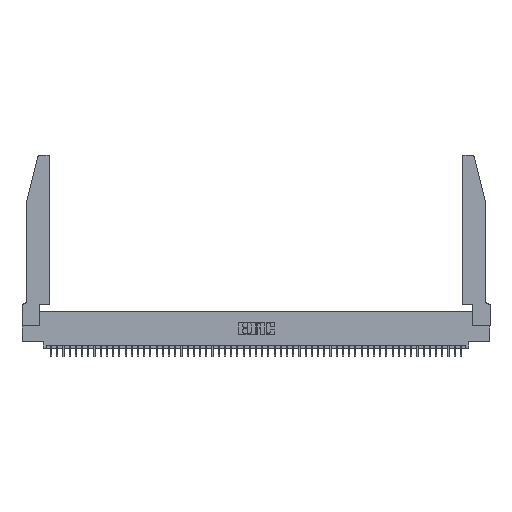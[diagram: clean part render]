
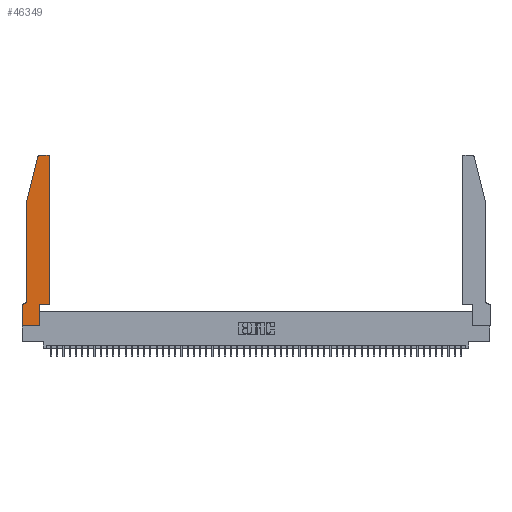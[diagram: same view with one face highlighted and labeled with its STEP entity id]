
A CAD part, top view. The second image highlights one B-rep face of the part: STEP entity #46349.
In plain terms, the highlighted planar face has unit normal (0, 0, 1).
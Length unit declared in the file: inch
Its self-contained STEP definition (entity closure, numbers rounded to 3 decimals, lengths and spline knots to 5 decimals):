
#255 = EDGE_CURVE ( 'NONE', #29158, #11118, #25259, .T. ) ;
#422 = DIRECTION ( 'NONE',  ( 0., 1., 0. ) ) ;
#855 = CARTESIAN_POINT ( 'NONE',  ( 0., 0.35, 0.37 ) ) ;
#1293 = VECTOR ( 'NONE', #41936, 39.37008 ) ;
#1744 = LINE ( 'NONE', #14056, #22702 ) ;
#2047 = ORIENTED_EDGE ( 'NONE', *, *, #10825, .T. ) ;
#2261 = VECTOR ( 'NONE', #49794, 39.37008 ) ;
#2536 = EDGE_CURVE ( 'NONE', #11118, #16320, #14779, .T. ) ;
#3194 = LINE ( 'NONE', #44871, #2261 ) ;
#4353 = VERTEX_POINT ( 'NONE', #20992 ) ;
#4741 = DIRECTION ( 'NONE',  ( 1., 0., 0. ) ) ;
#5598 = LINE ( 'NONE', #26940, #16897 ) ;
#6244 = LINE ( 'NONE', #31736, #15475 ) ;
#6342 = AXIS2_PLACEMENT_3D ( 'NONE', #29683, #42881, #47290 ) ;
#6368 = EDGE_CURVE ( 'NONE', #54025, #15663, #5598, .T. ) ;
#8783 = CARTESIAN_POINT ( 'NONE',  ( 0.2605, 2.75, 0.37 ) ) ;
#10032 = CARTESIAN_POINT ( 'NONE',  ( 0., 0.35, 0.37 ) ) ;
#10690 = AXIS2_PLACEMENT_3D ( 'NONE', #32336, #24099, #11267 ) ;
#10755 = CIRCLE ( 'NONE', #6342, 0.03 ) ;
#10825 = EDGE_CURVE ( 'NONE', #53074, #42692, #49253, .T. ) ;
#10941 = CARTESIAN_POINT ( 'NONE',  ( 0.0755, 0.42, 0.37 ) ) ;
#11118 = VERTEX_POINT ( 'NONE', #38383 ) ;
#11267 = DIRECTION ( 'NONE',  ( 1., 0., 0. ) ) ;
#11764 = ORIENTED_EDGE ( 'NONE', *, *, #50175, .T. ) ;
#12223 = CARTESIAN_POINT ( 'NONE',  ( 0.0755, 0.35, 0.37 ) ) ;
#13361 = VECTOR ( 'NONE', #422, 39.37008 ) ;
#13656 = ORIENTED_EDGE ( 'NONE', *, *, #39989, .T. ) ;
#13779 = DIRECTION ( 'NONE',  ( 0., -1., 0. ) ) ;
#14056 = CARTESIAN_POINT ( 'NONE',  ( 0.0755, 2., 0.37 ) ) ;
#14239 = CARTESIAN_POINT ( 'NONE',  ( 0.4505, 0.35, 0.37 ) ) ;
#14523 = EDGE_CURVE ( 'NONE', #15663, #51088, #3194, .T. ) ;
#14779 = LINE ( 'NONE', #14239, #26258 ) ;
#14914 = PLANE ( 'NONE',  #29344 ) ;
#15116 = DIRECTION ( 'NONE',  ( 0., 0., -1. ) ) ;
#15122 = CARTESIAN_POINT ( 'NONE',  ( 0.284, 2.75, 0.37 ) ) ;
#15475 = VECTOR ( 'NONE', #23750, 39.37008 ) ;
#15663 = VERTEX_POINT ( 'NONE', #17989 ) ;
#16306 = CARTESIAN_POINT ( 'NONE',  ( 0.0055, 0.35, 0.37 ) ) ;
#16320 = VERTEX_POINT ( 'NONE', #30706 ) ;
#16897 = VECTOR ( 'NONE', #27759, 39.37008 ) ;
#17989 = CARTESIAN_POINT ( 'NONE',  ( 0., 0., 0.37 ) ) ;
#19514 = VERTEX_POINT ( 'NONE', #15122 ) ;
#20992 = CARTESIAN_POINT ( 'NONE',  ( 0.0755, 2., 0.37 ) ) ;
#22702 = VECTOR ( 'NONE', #13779, 39.37008 ) ;
#22761 = EDGE_CURVE ( 'NONE', #16320, #41802, #10755, .T. ) ;
#23306 = CARTESIAN_POINT ( 'NONE',  ( 0.0055, 0.42, 0.37 ) ) ;
#23750 = DIRECTION ( 'NONE',  ( -0.239, -0.971, 0. ) ) ;
#24099 = DIRECTION ( 'NONE',  ( 0., 0., 1. ) ) ;
#25153 = EDGE_CURVE ( 'NONE', #51088, #29158, #49566, .T. ) ;
#25259 = LINE ( 'NONE', #51108, #38154 ) ;
#25531 = AXIS2_PLACEMENT_3D ( 'NONE', #23306, #15116, #40077 ) ;
#25700 = CARTESIAN_POINT ( 'NONE',  ( 0.25487, 2.72718, 0.37 ) ) ;
#26041 = ORIENTED_EDGE ( 'NONE', *, *, #22761, .T. ) ;
#26258 = VECTOR ( 'NONE', #43601, 39.37008 ) ;
#26940 = CARTESIAN_POINT ( 'NONE',  ( 0., 0., 0.37 ) ) ;
#27759 = DIRECTION ( 'NONE',  ( 0., -1., 0. ) ) ;
#28499 = CARTESIAN_POINT ( 'NONE',  ( 0.2865, 0., 0.37 ) ) ;
#29158 = VERTEX_POINT ( 'NONE', #41702 ) ;
#29344 = AXIS2_PLACEMENT_3D ( 'NONE', #10032, #30525, #47316 ) ;
#29519 = ORIENTED_EDGE ( 'NONE', *, *, #25153, .T. ) ;
#29683 = CARTESIAN_POINT ( 'NONE',  ( 0.4205, 2.72, 0.37 ) ) ;
#30089 = VECTOR ( 'NONE', #45693, 39.37008 ) ;
#30525 = DIRECTION ( 'NONE',  ( 0., 0., 1. ) ) ;
#30706 = CARTESIAN_POINT ( 'NONE',  ( 0.4505, 2.72, 0.37 ) ) ;
#31736 = CARTESIAN_POINT ( 'NONE',  ( 0.0755, 2., 0.37 ) ) ;
#32336 = CARTESIAN_POINT ( 'NONE',  ( 0.284, 2.72, 0.37 ) ) ;
#32991 = CARTESIAN_POINT ( 'NONE',  ( 0.4205, 2.75, 0.37 ) ) ;
#34286 = CIRCLE ( 'NONE', #10690, 0.03 ) ;
#35895 = EDGE_CURVE ( 'NONE', #4353, #53074, #1744, .T. ) ;
#36935 = CARTESIAN_POINT ( 'NONE',  ( 0.2865, 0.35, 0.37 ) ) ;
#38154 = VECTOR ( 'NONE', #4741, 39.37008 ) ;
#38383 = CARTESIAN_POINT ( 'NONE',  ( 0.4505, 0.35, 0.37 ) ) ;
#39989 = EDGE_CURVE ( 'NONE', #19514, #40177, #34286, .T. ) ;
#40077 = DIRECTION ( 'NONE',  ( -1., 0., 0. ) ) ;
#40177 = VERTEX_POINT ( 'NONE', #25700 ) ;
#41702 = CARTESIAN_POINT ( 'NONE',  ( 0.2865, 0.35, 0.37 ) ) ;
#41766 = ORIENTED_EDGE ( 'NONE', *, *, #6368, .T. ) ;
#41802 = VERTEX_POINT ( 'NONE', #32991 ) ;
#41936 = DIRECTION ( 'NONE',  ( -1., 0., 0. ) ) ;
#42083 = LINE ( 'NONE', #12223, #30089 ) ;
#42284 = ORIENTED_EDGE ( 'NONE', *, *, #45264, .T. ) ;
#42692 = VERTEX_POINT ( 'NONE', #16306 ) ;
#42881 = DIRECTION ( 'NONE',  ( 0., 0., 1. ) ) ;
#42897 = ORIENTED_EDGE ( 'NONE', *, *, #255, .T. ) ;
#43601 = DIRECTION ( 'NONE',  ( 0., 1., 0. ) ) ;
#44871 = CARTESIAN_POINT ( 'NONE',  ( 0., 0., 0.37 ) ) ;
#44894 = ORIENTED_EDGE ( 'NONE', *, *, #53060, .T. ) ;
#45264 = EDGE_CURVE ( 'NONE', #41802, #19514, #47176, .T. ) ;
#45611 = ORIENTED_EDGE ( 'NONE', *, *, #14523, .T. ) ;
#45693 = DIRECTION ( 'NONE',  ( -1., 0., 0. ) ) ;
#46349 = ADVANCED_FACE ( 'NONE', ( #52506 ), #14914, .T. ) ;
#47176 = LINE ( 'NONE', #8783, #1293 ) ;
#47290 = DIRECTION ( 'NONE',  ( 1., 0., 0. ) ) ;
#47316 = DIRECTION ( 'NONE',  ( 1., 0., 0. ) ) ;
#47483 = ORIENTED_EDGE ( 'NONE', *, *, #2536, .T. ) ;
#49253 = CIRCLE ( 'NONE', #25531, 0.07 ) ;
#49566 = LINE ( 'NONE', #36935, #13361 ) ;
#49794 = DIRECTION ( 'NONE',  ( 1., 0., 0. ) ) ;
#50175 = EDGE_CURVE ( 'NONE', #42692, #54025, #42083, .T. ) ;
#51088 = VERTEX_POINT ( 'NONE', #28499 ) ;
#51108 = CARTESIAN_POINT ( 'NONE',  ( 0.4505, 0.35, 0.37 ) ) ;
#51651 = ORIENTED_EDGE ( 'NONE', *, *, #35895, .T. ) ;
#51799 = EDGE_LOOP ( 'NONE', ( #42284, #13656, #44894, #51651, #2047, #11764, #41766, #45611, #29519, #42897, #47483, #26041 ) ) ;
#52506 = FACE_OUTER_BOUND ( 'NONE', #51799, .T. ) ;
#53060 = EDGE_CURVE ( 'NONE', #40177, #4353, #6244, .T. ) ;
#53074 = VERTEX_POINT ( 'NONE', #10941 ) ;
#54025 = VERTEX_POINT ( 'NONE', #855 ) ;
